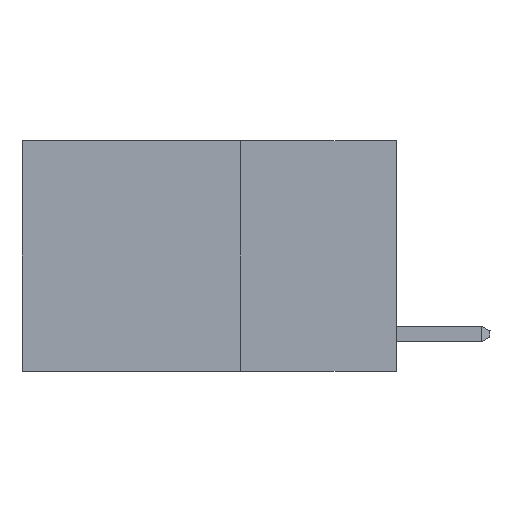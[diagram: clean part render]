
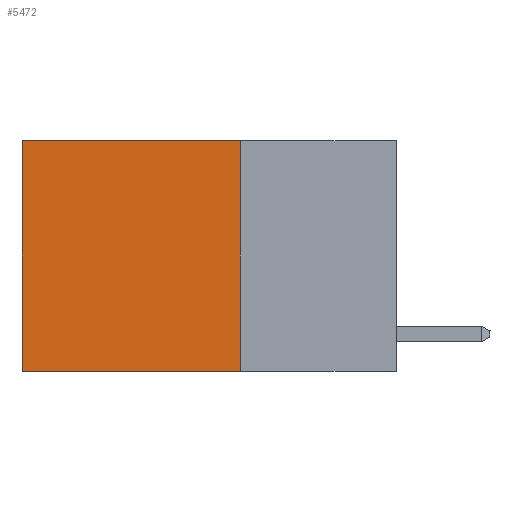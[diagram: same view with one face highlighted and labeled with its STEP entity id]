
A CAD part, left-side view. The second image highlights one B-rep face of the part: STEP entity #5472.
In plain terms, the highlighted planar face has unit normal (-1, 0, 0).
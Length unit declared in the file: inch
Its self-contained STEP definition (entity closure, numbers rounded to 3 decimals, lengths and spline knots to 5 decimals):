
#60 = DIRECTION ( 'NONE',  ( 0., 1., 0. ) ) ;
#269 = CARTESIAN_POINT ( 'NONE',  ( 0.2625, 0.25, 0. ) ) ;
#416 = ORIENTED_EDGE ( 'NONE', *, *, #5785, .F. ) ;
#525 = LINE ( 'NONE', #269, #9784 ) ;
#1020 = DIRECTION ( 'NONE',  ( 0., 0., -1. ) ) ;
#1091 = LINE ( 'NONE', #5628, #1522 ) ;
#1297 = CARTESIAN_POINT ( 'NONE',  ( 0.2625, 0.6, 0. ) ) ;
#1522 = VECTOR ( 'NONE', #1020, 39.37008 ) ;
#2157 = ORIENTED_EDGE ( 'NONE', *, *, #5916, .T. ) ;
#2569 = CARTESIAN_POINT ( 'NONE',  ( 0.2625, 0.25, 0. ) ) ;
#2902 = EDGE_CURVE ( 'NONE', #6832, #10485, #10617, .T. ) ;
#3634 = ORIENTED_EDGE ( 'NONE', *, *, #2902, .F. ) ;
#4101 = PLANE ( 'NONE',  #4229 ) ;
#4229 = AXIS2_PLACEMENT_3D ( 'NONE', #10576, #11480, #10615 ) ;
#4586 = VECTOR ( 'NONE', #7692, 39.37008 ) ;
#4640 = CARTESIAN_POINT ( 'NONE',  ( 0.2625, 0.25, -0.37 ) ) ;
#5472 = ADVANCED_FACE ( 'NONE', ( #6032 ), #4101, .F. ) ;
#5628 = CARTESIAN_POINT ( 'NONE',  ( 0.2625, 0.6, 0. ) ) ;
#5785 = EDGE_CURVE ( 'NONE', #7890, #6832, #8936, .T. ) ;
#5916 = EDGE_CURVE ( 'NONE', #10283, #10485, #1091, .T. ) ;
#6032 = FACE_OUTER_BOUND ( 'NONE', #11401, .T. ) ;
#6094 = DIRECTION ( 'NONE',  ( 0., 1., 0. ) ) ;
#6313 = EDGE_CURVE ( 'NONE', #7890, #10283, #525, .T. ) ;
#6832 = VERTEX_POINT ( 'NONE', #7972 ) ;
#7027 = ORIENTED_EDGE ( 'NONE', *, *, #6313, .T. ) ;
#7692 = DIRECTION ( 'NONE',  ( 0., 0., -1. ) ) ;
#7890 = VERTEX_POINT ( 'NONE', #2569 ) ;
#7972 = CARTESIAN_POINT ( 'NONE',  ( 0.2625, 0.25, -0.37 ) ) ;
#8936 = LINE ( 'NONE', #10823, #4586 ) ;
#9784 = VECTOR ( 'NONE', #6094, 39.37008 ) ;
#10283 = VERTEX_POINT ( 'NONE', #1297 ) ;
#10485 = VERTEX_POINT ( 'NONE', #10814 ) ;
#10576 = CARTESIAN_POINT ( 'NONE',  ( 0.2625, 0.25, 0. ) ) ;
#10615 = DIRECTION ( 'NONE',  ( 0., 0., -1. ) ) ;
#10617 = LINE ( 'NONE', #4640, #10747 ) ;
#10747 = VECTOR ( 'NONE', #60, 39.37008 ) ;
#10814 = CARTESIAN_POINT ( 'NONE',  ( 0.2625, 0.6, -0.37 ) ) ;
#10823 = CARTESIAN_POINT ( 'NONE',  ( 0.2625, 0.25, 0. ) ) ;
#11401 = EDGE_LOOP ( 'NONE', ( #2157, #3634, #416, #7027 ) ) ;
#11480 = DIRECTION ( 'NONE',  ( 1., 0., 0. ) ) ;
